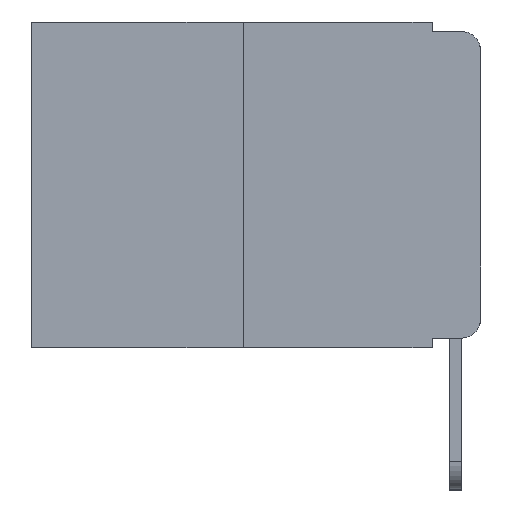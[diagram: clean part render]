
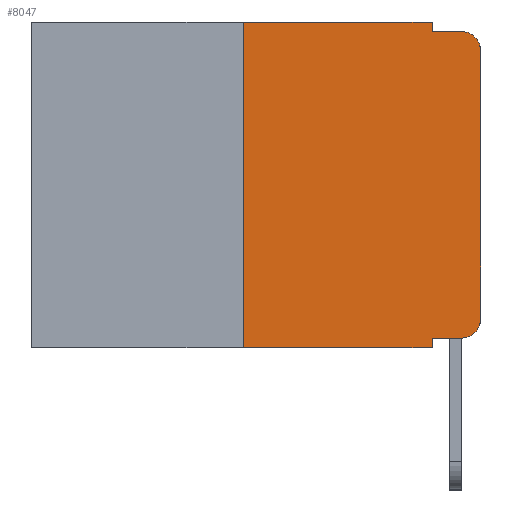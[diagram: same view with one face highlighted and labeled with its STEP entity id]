
A CAD part, left-side view. The second image highlights one B-rep face of the part: STEP entity #8047.
In plain terms, the highlighted planar face has unit normal (-1, 0, 0).
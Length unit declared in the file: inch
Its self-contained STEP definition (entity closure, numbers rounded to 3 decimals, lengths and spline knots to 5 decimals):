
#29 = EDGE_CURVE ( 'NONE', #6302, #11382, #15587, .T. ) ;
#30 = CARTESIAN_POINT ( 'NONE',  ( 0., 0.051, -0.333 ) ) ;
#323 = CARTESIAN_POINT ( 'NONE',  ( 0., 0.25, 0. ) ) ;
#448 = CARTESIAN_POINT ( 'NONE',  ( 0., 0.473, 0. ) ) ;
#885 = ORIENTED_EDGE ( 'NONE', *, *, #7049, .F. ) ;
#1173 = ORIENTED_EDGE ( 'NONE', *, *, #10888, .T. ) ;
#1255 = VERTEX_POINT ( 'NONE', #2778 ) ;
#1462 = CIRCLE ( 'NONE', #2906, 0.02 ) ;
#1667 = PLANE ( 'NONE',  #1790 ) ;
#1790 = AXIS2_PLACEMENT_3D ( 'NONE', #448, #10493, #14273 ) ;
#2168 = VECTOR ( 'NONE', #13388, 39.37008 ) ;
#2260 = EDGE_CURVE ( 'NONE', #13587, #9413, #2820, .T. ) ;
#2385 = LINE ( 'NONE', #14143, #15470 ) ;
#2514 = DIRECTION ( 'NONE',  ( 0., -1., 0. ) ) ;
#2778 = CARTESIAN_POINT ( 'NONE',  ( 0., 0., -0.03 ) ) ;
#2820 = LINE ( 'NONE', #15896, #11491 ) ;
#2906 = AXIS2_PLACEMENT_3D ( 'NONE', #5103, #9277, #13141 ) ;
#3157 = CARTESIAN_POINT ( 'NONE',  ( 0., 0.051, -0.333 ) ) ;
#3242 = VERTEX_POINT ( 'NONE', #3612 ) ;
#3548 = DIRECTION ( 'NONE',  ( 0., 0., -1. ) ) ;
#3612 = CARTESIAN_POINT ( 'NONE',  ( 0., 0.02, -0.01 ) ) ;
#4240 = CARTESIAN_POINT ( 'NONE',  ( 0., 0.02, -0.03 ) ) ;
#4359 = ORIENTED_EDGE ( 'NONE', *, *, #14800, .F. ) ;
#4646 = DIRECTION ( 'NONE',  ( 0., 0., -1. ) ) ;
#4818 = VERTEX_POINT ( 'NONE', #5477 ) ;
#4986 = CARTESIAN_POINT ( 'NONE',  ( 0., 0.25, -0.343 ) ) ;
#4994 = ORIENTED_EDGE ( 'NONE', *, *, #7571, .F. ) ;
#5103 = CARTESIAN_POINT ( 'NONE',  ( 0., 0.02, -0.313 ) ) ;
#5231 = LINE ( 'NONE', #15182, #12514 ) ;
#5477 = CARTESIAN_POINT ( 'NONE',  ( 0., 0.02, -0.333 ) ) ;
#5943 = FACE_OUTER_BOUND ( 'NONE', #14768, .T. ) ;
#6035 = CIRCLE ( 'NONE', #7034, 0.02 ) ;
#6302 = VERTEX_POINT ( 'NONE', #4986 ) ;
#6625 = DIRECTION ( 'NONE',  ( 0., -1., 0. ) ) ;
#6755 = ORIENTED_EDGE ( 'NONE', *, *, #2260, .F. ) ;
#7034 = AXIS2_PLACEMENT_3D ( 'NONE', #4240, #14412, #15644 ) ;
#7049 = EDGE_CURVE ( 'NONE', #6302, #14048, #13659, .T. ) ;
#7061 = CARTESIAN_POINT ( 'NONE',  ( 0., 0., 0. ) ) ;
#7561 = CARTESIAN_POINT ( 'NONE',  ( 0., 0., -0.313 ) ) ;
#7571 = EDGE_CURVE ( 'NONE', #14048, #13587, #2385, .T. ) ;
#7587 = DIRECTION ( 'NONE',  ( 0., -1., 0. ) ) ;
#7841 = ORIENTED_EDGE ( 'NONE', *, *, #29, .T. ) ;
#8047 = ADVANCED_FACE ( 'NONE', ( #5943 ), #1667, .F. ) ;
#8734 = EDGE_CURVE ( 'NONE', #13543, #1255, #11841, .T. ) ;
#9277 = DIRECTION ( 'NONE',  ( -1., 0., 0. ) ) ;
#9413 = VERTEX_POINT ( 'NONE', #9729 ) ;
#9521 = CARTESIAN_POINT ( 'NONE',  ( 0., 0.051, -0.343 ) ) ;
#9729 = CARTESIAN_POINT ( 'NONE',  ( 0., 0.051, -0.01 ) ) ;
#10416 = CARTESIAN_POINT ( 'NONE',  ( 0., 0.473, -0.343 ) ) ;
#10493 = DIRECTION ( 'NONE',  ( 1., 0., 0. ) ) ;
#10872 = LINE ( 'NONE', #11096, #15255 ) ;
#10888 = EDGE_CURVE ( 'NONE', #15200, #4818, #13540, .T. ) ;
#11012 = ORIENTED_EDGE ( 'NONE', *, *, #11199, .T. ) ;
#11096 = CARTESIAN_POINT ( 'NONE',  ( 0., 0.051, 0. ) ) ;
#11199 = EDGE_CURVE ( 'NONE', #1255, #3242, #6035, .T. ) ;
#11359 = VECTOR ( 'NONE', #2514, 39.37008 ) ;
#11382 = VERTEX_POINT ( 'NONE', #9521 ) ;
#11491 = VECTOR ( 'NONE', #4646, 39.37008 ) ;
#11636 = EDGE_CURVE ( 'NONE', #9413, #3242, #5231, .T. ) ;
#11841 = LINE ( 'NONE', #7061, #2168 ) ;
#11856 = ORIENTED_EDGE ( 'NONE', *, *, #11636, .F. ) ;
#12229 = CARTESIAN_POINT ( 'NONE',  ( 0., 0.051, 0. ) ) ;
#12514 = VECTOR ( 'NONE', #7587, 39.37008 ) ;
#13141 = DIRECTION ( 'NONE',  ( 0., 0., -1. ) ) ;
#13188 = DIRECTION ( 'NONE',  ( 0., 0., 1. ) ) ;
#13248 = EDGE_CURVE ( 'NONE', #4818, #13543, #1462, .T. ) ;
#13388 = DIRECTION ( 'NONE',  ( 0., 0., 1. ) ) ;
#13540 = LINE ( 'NONE', #30, #11359 ) ;
#13543 = VERTEX_POINT ( 'NONE', #7561 ) ;
#13587 = VERTEX_POINT ( 'NONE', #12229 ) ;
#13659 = LINE ( 'NONE', #323, #16280 ) ;
#13915 = DIRECTION ( 'NONE',  ( 0., -1., 0. ) ) ;
#14048 = VERTEX_POINT ( 'NONE', #16245 ) ;
#14143 = CARTESIAN_POINT ( 'NONE',  ( 0., 0.473, 0. ) ) ;
#14273 = DIRECTION ( 'NONE',  ( 0., 0., -1. ) ) ;
#14412 = DIRECTION ( 'NONE',  ( -1., 0., 0. ) ) ;
#14549 = ORIENTED_EDGE ( 'NONE', *, *, #13248, .T. ) ;
#14768 = EDGE_LOOP ( 'NONE', ( #15023, #11012, #11856, #6755, #4994, #885, #7841, #4359, #1173, #14549 ) ) ;
#14800 = EDGE_CURVE ( 'NONE', #15200, #11382, #10872, .T. ) ;
#15023 = ORIENTED_EDGE ( 'NONE', *, *, #8734, .T. ) ;
#15182 = CARTESIAN_POINT ( 'NONE',  ( 0., 0.051, -0.01 ) ) ;
#15183 = VECTOR ( 'NONE', #13915, 39.37008 ) ;
#15200 = VERTEX_POINT ( 'NONE', #3157 ) ;
#15255 = VECTOR ( 'NONE', #3548, 39.37008 ) ;
#15470 = VECTOR ( 'NONE', #6625, 39.37008 ) ;
#15587 = LINE ( 'NONE', #10416, #15183 ) ;
#15644 = DIRECTION ( 'NONE',  ( 0., 0., -1. ) ) ;
#15896 = CARTESIAN_POINT ( 'NONE',  ( 0., 0.051, 0. ) ) ;
#16245 = CARTESIAN_POINT ( 'NONE',  ( 0., 0.25, 0. ) ) ;
#16280 = VECTOR ( 'NONE', #13188, 39.37008 ) ;
